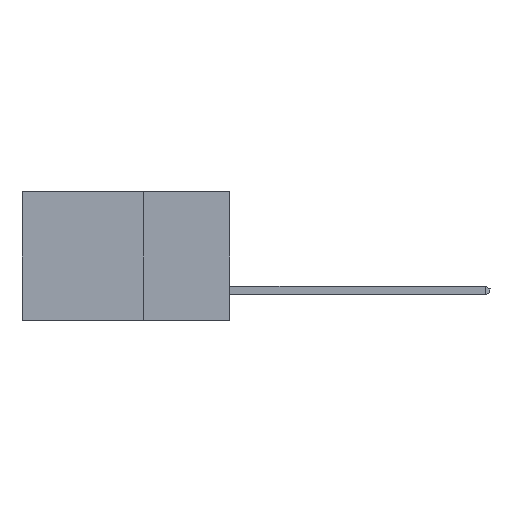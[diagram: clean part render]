
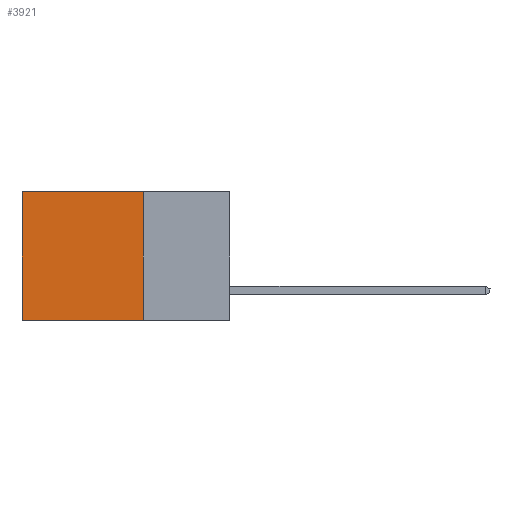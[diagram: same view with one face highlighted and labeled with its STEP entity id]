
A CAD part, left-side view. The second image highlights one B-rep face of the part: STEP entity #3921.
In plain terms, the highlighted planar face has unit normal (-1, 0, 0).
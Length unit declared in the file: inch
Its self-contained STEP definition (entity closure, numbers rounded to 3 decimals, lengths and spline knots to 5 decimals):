
#352 = CARTESIAN_POINT ( 'NONE',  ( 0.2615, 0.25, -0.37 ) ) ;
#1002 = DIRECTION ( 'NONE',  ( 1., 0., 0. ) ) ;
#1159 = CARTESIAN_POINT ( 'NONE',  ( 0.2615, 0.6, 0. ) ) ;
#1339 = LINE ( 'NONE', #3902, #11390 ) ;
#1471 = ORIENTED_EDGE ( 'NONE', *, *, #2450, .T. ) ;
#1601 = LINE ( 'NONE', #15516, #12345 ) ;
#2450 = EDGE_CURVE ( 'NONE', #15778, #4421, #11314, .T. ) ;
#2991 = CARTESIAN_POINT ( 'NONE',  ( 0.2615, 0.25, 0. ) ) ;
#3564 = CARTESIAN_POINT ( 'NONE',  ( 0.2615, 0.25, -0.37 ) ) ;
#3902 = CARTESIAN_POINT ( 'NONE',  ( 0.2615, 0.6, -0.37 ) ) ;
#3921 = ADVANCED_FACE ( 'NONE', ( #10478 ), #16025, .F. ) ;
#4421 = VERTEX_POINT ( 'NONE', #1159 ) ;
#4562 = CARTESIAN_POINT ( 'NONE',  ( 0.2615, 0.25, 0. ) ) ;
#5169 = EDGE_CURVE ( 'NONE', #16575, #5518, #1601, .T. ) ;
#5328 = ORIENTED_EDGE ( 'NONE', *, *, #15611, .T. ) ;
#5518 = VERTEX_POINT ( 'NONE', #15585 ) ;
#7081 = ORIENTED_EDGE ( 'NONE', *, *, #13561, .F. ) ;
#7277 = VECTOR ( 'NONE', #8937, 39.37008 ) ;
#8358 = DIRECTION ( 'NONE',  ( 0., 0., -1. ) ) ;
#8851 = CARTESIAN_POINT ( 'NONE',  ( 0.2615, 0.25, -0.37 ) ) ;
#8937 = DIRECTION ( 'NONE',  ( 0., 0., -1. ) ) ;
#9436 = EDGE_LOOP ( 'NONE', ( #5328, #12647, #7081, #1471 ) ) ;
#10206 = DIRECTION ( 'NONE',  ( 0., 1., 0. ) ) ;
#10478 = FACE_OUTER_BOUND ( 'NONE', #9436, .T. ) ;
#11014 = AXIS2_PLACEMENT_3D ( 'NONE', #3564, #1002, #14734 ) ;
#11314 = LINE ( 'NONE', #4562, #15079 ) ;
#11390 = VECTOR ( 'NONE', #8358, 39.37008 ) ;
#12345 = VECTOR ( 'NONE', #12510, 39.37008 ) ;
#12510 = DIRECTION ( 'NONE',  ( 0., 1., 0. ) ) ;
#12647 = ORIENTED_EDGE ( 'NONE', *, *, #5169, .F. ) ;
#13561 = EDGE_CURVE ( 'NONE', #15778, #16575, #15853, .T. ) ;
#14734 = DIRECTION ( 'NONE',  ( 0., 0., -1. ) ) ;
#15079 = VECTOR ( 'NONE', #10206, 39.37008 ) ;
#15516 = CARTESIAN_POINT ( 'NONE',  ( 0.2615, 0.25, -0.37 ) ) ;
#15585 = CARTESIAN_POINT ( 'NONE',  ( 0.2615, 0.6, -0.37 ) ) ;
#15611 = EDGE_CURVE ( 'NONE', #4421, #5518, #1339, .T. ) ;
#15778 = VERTEX_POINT ( 'NONE', #2991 ) ;
#15853 = LINE ( 'NONE', #8851, #7277 ) ;
#16025 = PLANE ( 'NONE',  #11014 ) ;
#16575 = VERTEX_POINT ( 'NONE', #352 ) ;
